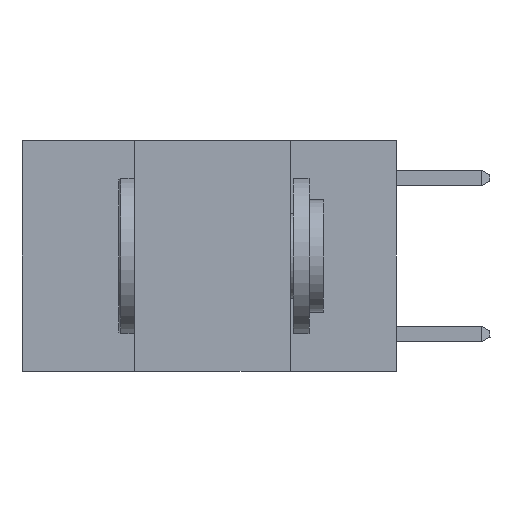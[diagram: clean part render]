
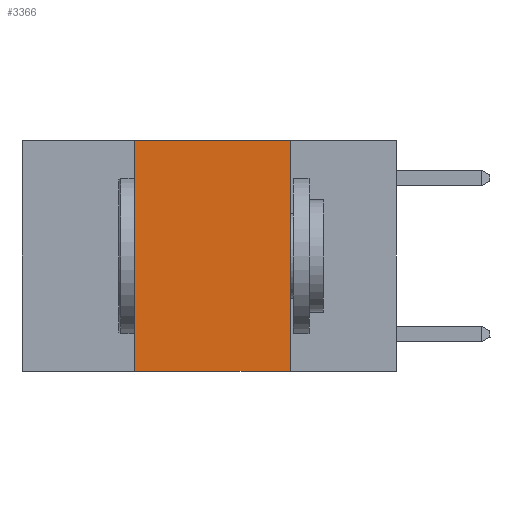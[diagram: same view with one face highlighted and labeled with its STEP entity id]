
A CAD part, left-side view. The second image highlights one B-rep face of the part: STEP entity #3366.
In plain terms, the highlighted planar face has unit normal (-1, 0, 0).
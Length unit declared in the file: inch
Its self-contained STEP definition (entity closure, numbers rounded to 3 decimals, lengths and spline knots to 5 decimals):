
#168 = VERTEX_POINT ( 'NONE', #2996 ) ;
#688 = DIRECTION ( 'NONE',  ( 0., 0., -1. ) ) ;
#1838 = CARTESIAN_POINT ( 'NONE',  ( 0., 0.17, 0. ) ) ;
#2723 = CARTESIAN_POINT ( 'NONE',  ( 0., 0.6, 0. ) ) ;
#2963 = DIRECTION ( 'NONE',  ( 0., 0., 1. ) ) ;
#2996 = CARTESIAN_POINT ( 'NONE',  ( 0., 0.42, -0.37 ) ) ;
#3291 = CARTESIAN_POINT ( 'NONE',  ( 0., 0.6, -0.37 ) ) ;
#3366 = ADVANCED_FACE ( 'NONE', ( #11318 ), #5165, .F. ) ;
#3559 = ORIENTED_EDGE ( 'NONE', *, *, #7870, .T. ) ;
#3601 = VERTEX_POINT ( 'NONE', #8765 ) ;
#4052 = VECTOR ( 'NONE', #9054, 39.37008 ) ;
#4172 = LINE ( 'NONE', #3291, #7035 ) ;
#4353 = VECTOR ( 'NONE', #688, 39.37008 ) ;
#5165 = PLANE ( 'NONE',  #13335 ) ;
#5805 = EDGE_CURVE ( 'NONE', #12359, #3601, #9979, .T. ) ;
#6768 = CARTESIAN_POINT ( 'NONE',  ( 0., 0.42, 0. ) ) ;
#6798 = ORIENTED_EDGE ( 'NONE', *, *, #7608, .F. ) ;
#7035 = VECTOR ( 'NONE', #10640, 39.37008 ) ;
#7213 = LINE ( 'NONE', #7275, #12316 ) ;
#7275 = CARTESIAN_POINT ( 'NONE',  ( 0., 0.42, 0. ) ) ;
#7355 = DIRECTION ( 'NONE',  ( 0., 0., -1. ) ) ;
#7531 = LINE ( 'NONE', #1838, #4353 ) ;
#7588 = EDGE_CURVE ( 'NONE', #3601, #10015, #7531, .T. ) ;
#7608 = EDGE_CURVE ( 'NONE', #168, #12359, #7213, .T. ) ;
#7870 = EDGE_CURVE ( 'NONE', #168, #10015, #4172, .T. ) ;
#8564 = ORIENTED_EDGE ( 'NONE', *, *, #7588, .F. ) ;
#8765 = CARTESIAN_POINT ( 'NONE',  ( 0., 0.17, 0. ) ) ;
#9054 = DIRECTION ( 'NONE',  ( 0., -1., 0. ) ) ;
#9373 = CARTESIAN_POINT ( 'NONE',  ( 0., 0.6, 0. ) ) ;
#9979 = LINE ( 'NONE', #2723, #4052 ) ;
#10015 = VERTEX_POINT ( 'NONE', #12101 ) ;
#10640 = DIRECTION ( 'NONE',  ( 0., -1., 0. ) ) ;
#10713 = EDGE_LOOP ( 'NONE', ( #8564, #11282, #6798, #3559 ) ) ;
#11282 = ORIENTED_EDGE ( 'NONE', *, *, #5805, .F. ) ;
#11318 = FACE_OUTER_BOUND ( 'NONE', #10713, .T. ) ;
#12101 = CARTESIAN_POINT ( 'NONE',  ( 0., 0.17, -0.37 ) ) ;
#12316 = VECTOR ( 'NONE', #2963, 39.37008 ) ;
#12359 = VERTEX_POINT ( 'NONE', #6768 ) ;
#13335 = AXIS2_PLACEMENT_3D ( 'NONE', #9373, #13440, #7355 ) ;
#13440 = DIRECTION ( 'NONE',  ( 1., 0., 0. ) ) ;
